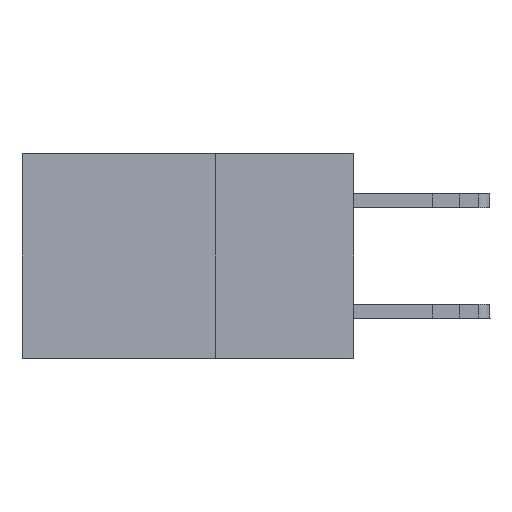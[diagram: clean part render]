
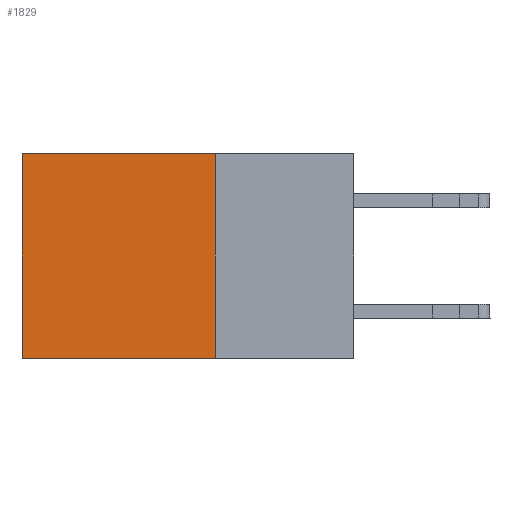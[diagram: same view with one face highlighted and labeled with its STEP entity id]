
A CAD part, left-side view. The second image highlights one B-rep face of the part: STEP entity #1829.
In plain terms, the highlighted planar face has unit normal (-1, 0, 0).
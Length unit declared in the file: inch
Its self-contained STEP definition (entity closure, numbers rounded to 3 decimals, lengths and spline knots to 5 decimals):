
#111 = PLANE ( 'NONE',  #4543 ) ;
#210 = ORIENTED_EDGE ( 'NONE', *, *, #8178, .T. ) ;
#365 = LINE ( 'NONE', #5319, #7247 ) ;
#1165 = CARTESIAN_POINT ( 'NONE',  ( 0.2875, 0.6, 0. ) ) ;
#1398 = LINE ( 'NONE', #12239, #2079 ) ;
#1821 = VERTEX_POINT ( 'NONE', #9850 ) ;
#1829 = ADVANCED_FACE ( 'NONE', ( #6132 ), #111, .F. ) ;
#2079 = VECTOR ( 'NONE', #12399, 39.37008 ) ;
#2787 = VERTEX_POINT ( 'NONE', #9012 ) ;
#3080 = VECTOR ( 'NONE', #11961, 39.37008 ) ;
#3370 = ORIENTED_EDGE ( 'NONE', *, *, #7914, .T. ) ;
#3807 = EDGE_CURVE ( 'NONE', #2787, #5287, #1398, .T. ) ;
#4447 = VECTOR ( 'NONE', #15686, 39.37008 ) ;
#4543 = AXIS2_PLACEMENT_3D ( 'NONE', #14788, #8805, #6217 ) ;
#4826 = LINE ( 'NONE', #1165, #3080 ) ;
#4858 = LINE ( 'NONE', #15774, #4447 ) ;
#5287 = VERTEX_POINT ( 'NONE', #13079 ) ;
#5319 = CARTESIAN_POINT ( 'NONE',  ( 0.2875, 0.25, 0. ) ) ;
#5687 = VERTEX_POINT ( 'NONE', #12917 ) ;
#6132 = FACE_OUTER_BOUND ( 'NONE', #10820, .T. ) ;
#6217 = DIRECTION ( 'NONE',  ( 0., 0., -1. ) ) ;
#7247 = VECTOR ( 'NONE', #10249, 39.37008 ) ;
#7914 = EDGE_CURVE ( 'NONE', #1821, #5687, #4826, .T. ) ;
#8178 = EDGE_CURVE ( 'NONE', #2787, #1821, #365, .T. ) ;
#8805 = DIRECTION ( 'NONE',  ( 1., 0., 0. ) ) ;
#9012 = CARTESIAN_POINT ( 'NONE',  ( 0.2875, 0.25, 0. ) ) ;
#9850 = CARTESIAN_POINT ( 'NONE',  ( 0.2875, 0.6, 0. ) ) ;
#10249 = DIRECTION ( 'NONE',  ( 0., 1., 0. ) ) ;
#10820 = EDGE_LOOP ( 'NONE', ( #3370, #11846, #12572, #210 ) ) ;
#11846 = ORIENTED_EDGE ( 'NONE', *, *, #15868, .F. ) ;
#11961 = DIRECTION ( 'NONE',  ( 0., 0., -1. ) ) ;
#12239 = CARTESIAN_POINT ( 'NONE',  ( 0.2875, 0.25, 0. ) ) ;
#12399 = DIRECTION ( 'NONE',  ( 0., 0., -1. ) ) ;
#12572 = ORIENTED_EDGE ( 'NONE', *, *, #3807, .F. ) ;
#12917 = CARTESIAN_POINT ( 'NONE',  ( 0.2875, 0.6, -0.37 ) ) ;
#13079 = CARTESIAN_POINT ( 'NONE',  ( 0.2875, 0.25, -0.37 ) ) ;
#14788 = CARTESIAN_POINT ( 'NONE',  ( 0.2875, 0.25, 0. ) ) ;
#15686 = DIRECTION ( 'NONE',  ( 0., 1., 0. ) ) ;
#15774 = CARTESIAN_POINT ( 'NONE',  ( 0.2875, 0.25, -0.37 ) ) ;
#15868 = EDGE_CURVE ( 'NONE', #5287, #5687, #4858, .T. ) ;
